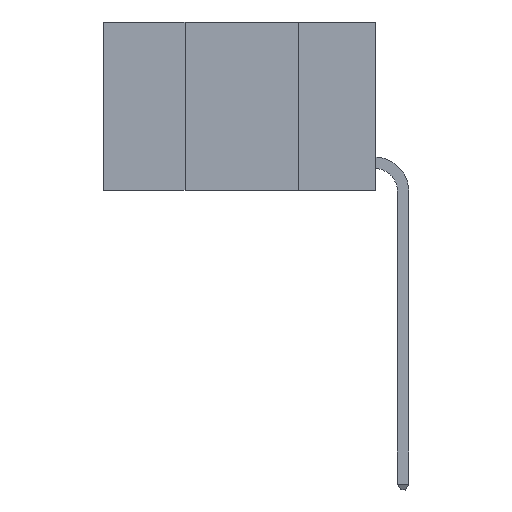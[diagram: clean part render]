
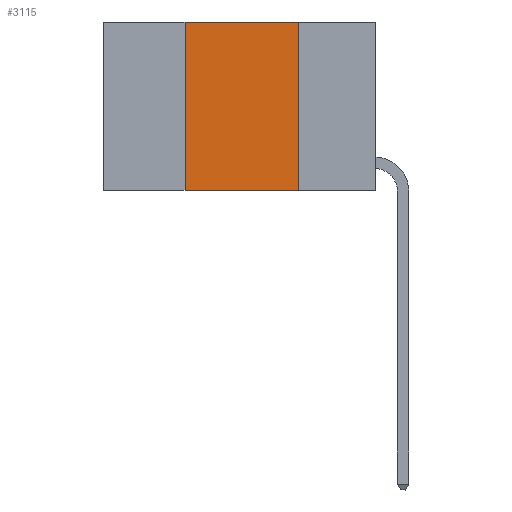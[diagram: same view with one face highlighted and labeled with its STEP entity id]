
A CAD part, left-side view. The second image highlights one B-rep face of the part: STEP entity #3115.
In plain terms, the highlighted planar face has unit normal (-1, 0, 0).
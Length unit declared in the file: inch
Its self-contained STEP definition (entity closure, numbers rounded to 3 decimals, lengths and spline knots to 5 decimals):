
#233 = CARTESIAN_POINT ( 'NONE',  ( 0., 0.17, -0.37 ) ) ;
#565 = EDGE_CURVE ( 'NONE', #8635, #8839, #2842, .T. ) ;
#653 = CARTESIAN_POINT ( 'NONE',  ( 0., 0.6, 0. ) ) ;
#1186 = EDGE_CURVE ( 'NONE', #8839, #6725, #11041, .T. ) ;
#1408 = CARTESIAN_POINT ( 'NONE',  ( 0., 0.17, 0. ) ) ;
#1670 = CARTESIAN_POINT ( 'NONE',  ( 0., 0.17, 0. ) ) ;
#2155 = AXIS2_PLACEMENT_3D ( 'NONE', #2730, #5751, #11743 ) ;
#2158 = EDGE_CURVE ( 'NONE', #5533, #8635, #8907, .T. ) ;
#2209 = EDGE_CURVE ( 'NONE', #5533, #6725, #5816, .T. ) ;
#2570 = EDGE_LOOP ( 'NONE', ( #9237, #7927, #7734, #11276 ) ) ;
#2730 = CARTESIAN_POINT ( 'NONE',  ( 0., 0.6, 0. ) ) ;
#2842 = LINE ( 'NONE', #653, #7545 ) ;
#3115 = ADVANCED_FACE ( 'NONE', ( #3861 ), #4828, .F. ) ;
#3861 = FACE_OUTER_BOUND ( 'NONE', #2570, .T. ) ;
#4018 = VECTOR ( 'NONE', #4019, 39.37008 ) ;
#4019 = DIRECTION ( 'NONE',  ( 0., 0., -1. ) ) ;
#4828 = PLANE ( 'NONE',  #2155 ) ;
#5489 = CARTESIAN_POINT ( 'NONE',  ( 0., 0.6, -0.37 ) ) ;
#5525 = DIRECTION ( 'NONE',  ( 0., -1., 0. ) ) ;
#5533 = VERTEX_POINT ( 'NONE', #9355 ) ;
#5751 = DIRECTION ( 'NONE',  ( 1., 0., 0. ) ) ;
#5816 = LINE ( 'NONE', #5489, #10120 ) ;
#6045 = DIRECTION ( 'NONE',  ( 0., -1., 0. ) ) ;
#6239 = DIRECTION ( 'NONE',  ( 0., 0., 1. ) ) ;
#6279 = CARTESIAN_POINT ( 'NONE',  ( 0., 0.42, 0. ) ) ;
#6651 = VECTOR ( 'NONE', #6239, 39.37008 ) ;
#6725 = VERTEX_POINT ( 'NONE', #233 ) ;
#7545 = VECTOR ( 'NONE', #6045, 39.37008 ) ;
#7734 = ORIENTED_EDGE ( 'NONE', *, *, #2158, .F. ) ;
#7927 = ORIENTED_EDGE ( 'NONE', *, *, #565, .F. ) ;
#8635 = VERTEX_POINT ( 'NONE', #12184 ) ;
#8839 = VERTEX_POINT ( 'NONE', #1408 ) ;
#8907 = LINE ( 'NONE', #6279, #6651 ) ;
#9237 = ORIENTED_EDGE ( 'NONE', *, *, #1186, .F. ) ;
#9355 = CARTESIAN_POINT ( 'NONE',  ( 0., 0.42, -0.37 ) ) ;
#10120 = VECTOR ( 'NONE', #5525, 39.37008 ) ;
#11041 = LINE ( 'NONE', #1670, #4018 ) ;
#11276 = ORIENTED_EDGE ( 'NONE', *, *, #2209, .T. ) ;
#11743 = DIRECTION ( 'NONE',  ( 0., 0., -1. ) ) ;
#12184 = CARTESIAN_POINT ( 'NONE',  ( 0., 0.42, 0. ) ) ;
